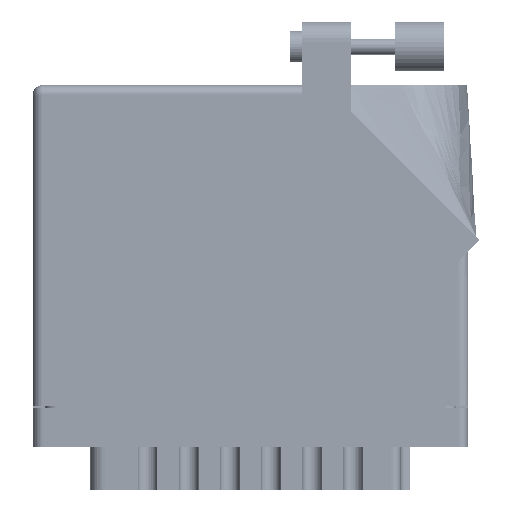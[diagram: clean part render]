
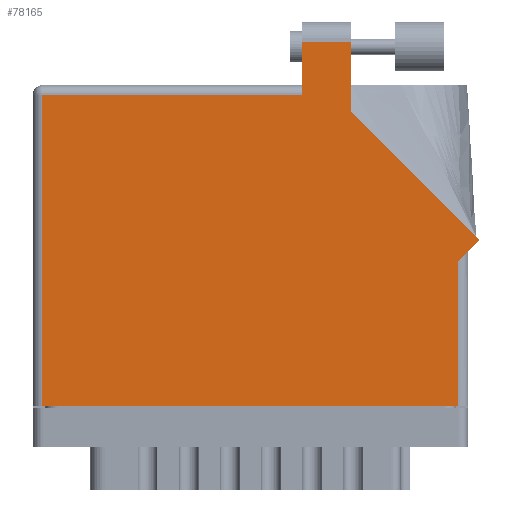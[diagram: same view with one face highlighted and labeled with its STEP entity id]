
A CAD part, front view. The second image highlights one B-rep face of the part: STEP entity #78165.
In plain terms, the highlighted face is planar.
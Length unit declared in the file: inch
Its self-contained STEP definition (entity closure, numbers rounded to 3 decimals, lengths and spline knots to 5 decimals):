
#708 = VECTOR ( 'NONE', #5702, 39.37008 ) ;
#743 = LINE ( 'NONE', #21313, #90518 ) ;
#1037 = ORIENTED_EDGE ( 'NONE', *, *, #13442, .T. ) ;
#2764 = FACE_OUTER_BOUND ( 'NONE', #13153, .T. ) ;
#4009 = LINE ( 'NONE', #42894, #47728 ) ;
#4888 = EDGE_CURVE ( 'NONE', #61978, #84086, #85310, .T. ) ;
#5702 = DIRECTION ( 'NONE',  ( 0., -1., 0. ) ) ;
#5743 = VERTEX_POINT ( 'NONE', #6850 ) ;
#5955 = ORIENTED_EDGE ( 'NONE', *, *, #88932, .T. ) ;
#6797 = LINE ( 'NONE', #55115, #80892 ) ;
#6825 = ORIENTED_EDGE ( 'NONE', *, *, #4888, .T. ) ;
#6850 = CARTESIAN_POINT ( 'NONE',  ( 1.705, 2.305, 0. ) ) ;
#6903 = CARTESIAN_POINT ( 'NONE',  ( 2.755, 0.98, 0. ) ) ;
#7239 = ORIENTED_EDGE ( 'NONE', *, *, #10615, .T. ) ;
#8069 = ORIENTED_EDGE ( 'NONE', *, *, #69307, .T. ) ;
#9589 = DIRECTION ( 'NONE',  ( 0., 1., 0. ) ) ;
#10615 = EDGE_CURVE ( 'NONE', #85063, #61978, #6797, .T. ) ;
#11114 = DIRECTION ( 'NONE',  ( 0., 1., 0. ) ) ;
#12130 = DIRECTION ( 'NONE',  ( -1., 0., 0. ) ) ;
#12291 = ORIENTED_EDGE ( 'NONE', *, *, #55613, .T. ) ;
#13153 = EDGE_LOOP ( 'NONE', ( #5955, #8069, #1037, #7239, #6825, #91985, #41383, #86433, #12291 ) ) ;
#13442 = EDGE_CURVE ( 'NONE', #5743, #85063, #43312, .T. ) ;
#15354 = CARTESIAN_POINT ( 'NONE',  ( 1.705, 1.968, 0. ) ) ;
#19781 = DIRECTION ( 'NONE',  ( -1., 0., 0. ) ) ;
#21313 = CARTESIAN_POINT ( 'NONE',  ( 2.82571, 1.05071, 0. ) ) ;
#23043 = VERTEX_POINT ( 'NONE', #26044 ) ;
#23926 = CARTESIAN_POINT ( 'NONE',  ( 0.062, 0., 0. ) ) ;
#26044 = CARTESIAN_POINT ( 'NONE',  ( 2.82571, 1.05071, 0. ) ) ;
#33324 = CARTESIAN_POINT ( 'NONE',  ( 0., 2.03, 0. ) ) ;
#35135 = DIRECTION ( 'NONE',  ( 0.707, 0.707, 0. ) ) ;
#37343 = VECTOR ( 'NONE', #9589, 39.37008 ) ;
#37457 = LINE ( 'NONE', #76068, #85720 ) ;
#41383 = ORIENTED_EDGE ( 'NONE', *, *, #43389, .T. ) ;
#42894 = CARTESIAN_POINT ( 'NONE',  ( 1.705, 2.305, 0. ) ) ;
#43312 = LINE ( 'NONE', #69405, #708 ) ;
#43389 = EDGE_CURVE ( 'NONE', #69121, #76130, #45163, .T. ) ;
#44175 = DIRECTION ( 'NONE',  ( -0.707, 0.707, 0. ) ) ;
#45163 = LINE ( 'NONE', #66405, #37343 ) ;
#45813 = CARTESIAN_POINT ( 'NONE',  ( 0., 0., 0. ) ) ;
#47728 = VECTOR ( 'NONE', #71795, 39.37008 ) ;
#51617 = CARTESIAN_POINT ( 'NONE',  ( 0.062, 1.968, 0. ) ) ;
#53130 = EDGE_CURVE ( 'NONE', #76130, #23043, #83632, .T. ) ;
#55115 = CARTESIAN_POINT ( 'NONE',  ( 0., 1.968, 0. ) ) ;
#55613 = EDGE_CURVE ( 'NONE', #23043, #80183, #743, .T. ) ;
#57610 = CARTESIAN_POINT ( 'NONE',  ( 2.012, 1.86442, 0. ) ) ;
#58375 = VECTOR ( 'NONE', #83560, 39.37008 ) ;
#58618 = VERTEX_POINT ( 'NONE', #80085 ) ;
#58658 = AXIS2_PLACEMENT_3D ( 'NONE', #33324, #76299, #19781 ) ;
#61083 = CARTESIAN_POINT ( 'NONE',  ( 0.062, 0., 0. ) ) ;
#61978 = VERTEX_POINT ( 'NONE', #51617 ) ;
#63082 = VECTOR ( 'NONE', #89761, 39.37008 ) ;
#64033 = CARTESIAN_POINT ( 'NONE',  ( 2.693, 0.918, 0. ) ) ;
#64528 = VECTOR ( 'NONE', #35135, 39.37008 ) ;
#65275 = EDGE_CURVE ( 'NONE', #84086, #69121, #72097, .T. ) ;
#66405 = CARTESIAN_POINT ( 'NONE',  ( 2.693, 0.98, 0. ) ) ;
#69121 = VERTEX_POINT ( 'NONE', #84998 ) ;
#69307 = EDGE_CURVE ( 'NONE', #58618, #5743, #4009, .T. ) ;
#69405 = CARTESIAN_POINT ( 'NONE',  ( 1.705, 2.03, 0. ) ) ;
#71795 = DIRECTION ( 'NONE',  ( -1., 0., 0. ) ) ;
#72097 = LINE ( 'NONE', #45813, #63082 ) ;
#76068 = CARTESIAN_POINT ( 'NONE',  ( 2.012, 1.86442, 0. ) ) ;
#76130 = VERTEX_POINT ( 'NONE', #64033 ) ;
#76299 = DIRECTION ( 'NONE',  ( 0., 0., -1. ) ) ;
#78165 = ADVANCED_FACE ( 'NONE', ( #2764 ), #83525, .F. ) ;
#80085 = CARTESIAN_POINT ( 'NONE',  ( 2.012, 2.305, 0. ) ) ;
#80183 = VERTEX_POINT ( 'NONE', #57610 ) ;
#80892 = VECTOR ( 'NONE', #12130, 39.37008 ) ;
#83525 = PLANE ( 'NONE',  #58658 ) ;
#83560 = DIRECTION ( 'NONE',  ( 0., -1., 0. ) ) ;
#83632 = LINE ( 'NONE', #6903, #64528 ) ;
#84086 = VERTEX_POINT ( 'NONE', #61083 ) ;
#84998 = CARTESIAN_POINT ( 'NONE',  ( 2.693, 0., 0. ) ) ;
#85063 = VERTEX_POINT ( 'NONE', #15354 ) ;
#85310 = LINE ( 'NONE', #23926, #58375 ) ;
#85720 = VECTOR ( 'NONE', #11114, 39.37008 ) ;
#86433 = ORIENTED_EDGE ( 'NONE', *, *, #53130, .T. ) ;
#88932 = EDGE_CURVE ( 'NONE', #80183, #58618, #37457, .T. ) ;
#89761 = DIRECTION ( 'NONE',  ( 1., 0., 0. ) ) ;
#90518 = VECTOR ( 'NONE', #44175, 39.37008 ) ;
#91985 = ORIENTED_EDGE ( 'NONE', *, *, #65275, .T. ) ;
